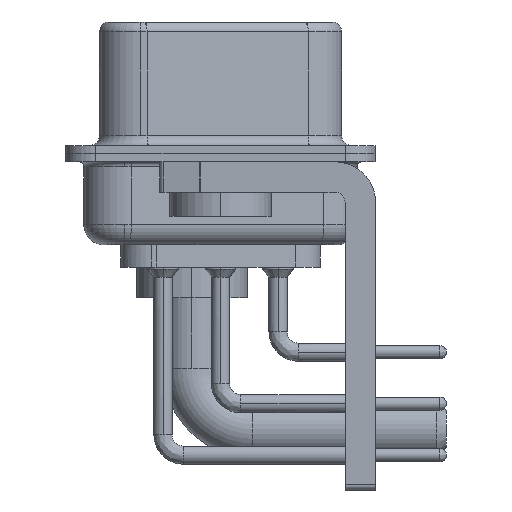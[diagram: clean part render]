
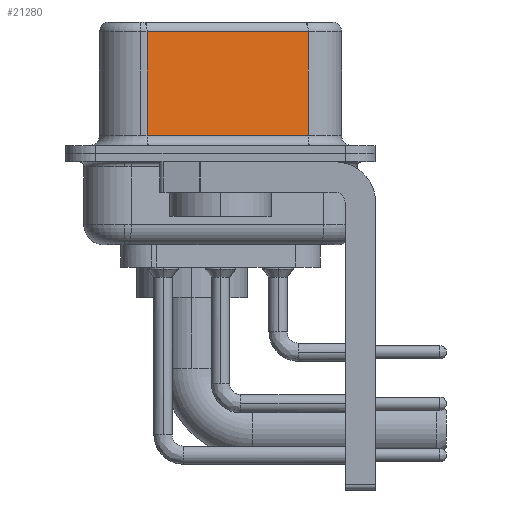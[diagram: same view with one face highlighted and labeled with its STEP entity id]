
A CAD part, left-side view. The second image highlights one B-rep face of the part: STEP entity #21280.
In plain terms, the highlighted planar face has unit normal (-0.985, -0.174, 0).
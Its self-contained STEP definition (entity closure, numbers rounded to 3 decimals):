
#1045 = DIRECTION ( 'NONE',  ( 0., 0., -1. ) ) ;
#1235 = EDGE_CURVE ( 'NONE', #37442, #30492, #5349, .T. ) ;
#2921 = CARTESIAN_POINT ( 'NONE',  ( 3.73, 3.628, 6.02 ) ) ;
#2988 = DIRECTION ( 'NONE',  ( 0.985, 0.174, 0. ) ) ;
#4955 = DIRECTION ( 'NONE',  ( 0., 0., -1. ) ) ;
#5227 = DIRECTION ( 'NONE',  ( -0.174, 0.985, 0. ) ) ;
#5349 = LINE ( 'NONE', #10974, #29389 ) ;
#5720 = FACE_OUTER_BOUND ( 'NONE', #37765, .T. ) ;
#5793 = VERTEX_POINT ( 'NONE', #8035 ) ;
#6088 = CARTESIAN_POINT ( 'NONE',  ( 3.73, 3.628, 6.52 ) ) ;
#8035 = CARTESIAN_POINT ( 'NONE',  ( 3.73, 3.628, 0.9 ) ) ;
#8148 = DIRECTION ( 'NONE',  ( 0.174, -0.985, 0. ) ) ;
#8339 = CARTESIAN_POINT ( 'NONE',  ( 5.132, -4.322, 0.9 ) ) ;
#9750 = LINE ( 'NONE', #6088, #22451 ) ;
#10974 = CARTESIAN_POINT ( 'NONE',  ( 5.132, -4.322, 6.52 ) ) ;
#11525 = EDGE_CURVE ( 'NONE', #28512, #5793, #9750, .T. ) ;
#11701 = DIRECTION ( 'NONE',  ( -0.174, 0.985, 0. ) ) ;
#15188 = PLANE ( 'NONE',  #29176 ) ;
#16240 = EDGE_CURVE ( 'NONE', #37442, #28512, #17614, .T. ) ;
#17614 = LINE ( 'NONE', #29458, #17967 ) ;
#17967 = VECTOR ( 'NONE', #5227, 1000. ) ;
#20063 = ORIENTED_EDGE ( 'NONE', *, *, #16240, .T. ) ;
#21280 = ADVANCED_FACE ( 'NONE', ( #5720 ), #15188, .F. ) ;
#21669 = ORIENTED_EDGE ( 'NONE', *, *, #34625, .T. ) ;
#22451 = VECTOR ( 'NONE', #1045, 1000. ) ;
#25809 = LINE ( 'NONE', #8339, #26483 ) ;
#26483 = VECTOR ( 'NONE', #8148, 1000. ) ;
#27027 = CARTESIAN_POINT ( 'NONE',  ( 5.132, -4.322, 6.52 ) ) ;
#28512 = VERTEX_POINT ( 'NONE', #2921 ) ;
#29090 = ORIENTED_EDGE ( 'NONE', *, *, #11525, .T. ) ;
#29176 = AXIS2_PLACEMENT_3D ( 'NONE', #27027, #2988, #11701 ) ;
#29389 = VECTOR ( 'NONE', #4955, 1000. ) ;
#29458 = CARTESIAN_POINT ( 'NONE',  ( 5.132, -4.322, 6.02 ) ) ;
#30279 = CARTESIAN_POINT ( 'NONE',  ( 5.132, -4.322, 6.02 ) ) ;
#30492 = VERTEX_POINT ( 'NONE', #34676 ) ;
#32979 = ORIENTED_EDGE ( 'NONE', *, *, #1235, .F. ) ;
#34625 = EDGE_CURVE ( 'NONE', #5793, #30492, #25809, .T. ) ;
#34676 = CARTESIAN_POINT ( 'NONE',  ( 5.132, -4.322, 0.9 ) ) ;
#37442 = VERTEX_POINT ( 'NONE', #30279 ) ;
#37765 = EDGE_LOOP ( 'NONE', ( #32979, #20063, #29090, #21669 ) ) ;
